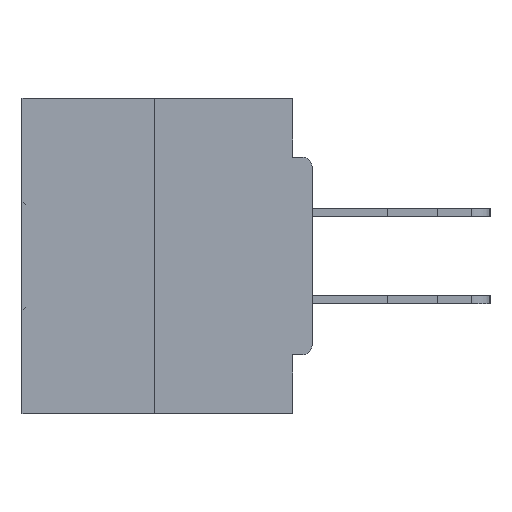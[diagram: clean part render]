
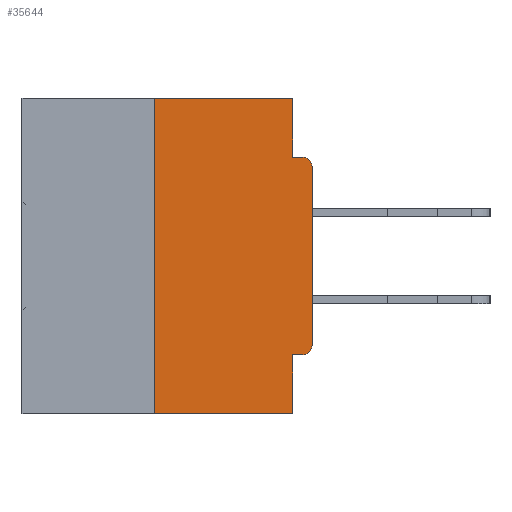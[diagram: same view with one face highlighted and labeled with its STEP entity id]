
A CAD part, left-side view. The second image highlights one B-rep face of the part: STEP entity #35644.
In plain terms, the highlighted planar face has unit normal (-1, 0, 0).
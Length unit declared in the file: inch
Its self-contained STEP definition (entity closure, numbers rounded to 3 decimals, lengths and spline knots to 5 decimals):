
#407 = VECTOR ( 'NONE', #23579, 39.37008 ) ;
#634 = DIRECTION ( 'NONE',  ( 1., 0., 0. ) ) ;
#1143 = EDGE_CURVE ( 'NONE', #27510, #11333, #8660, .T. ) ;
#1648 = CIRCLE ( 'NONE', #36667, 0.015 ) ;
#2024 = CARTESIAN_POINT ( 'NONE',  ( 0., 0.46, -0.5 ) ) ;
#2041 = ORIENTED_EDGE ( 'NONE', *, *, #32942, .F. ) ;
#2618 = VECTOR ( 'NONE', #38371, 39.37008 ) ;
#3004 = CARTESIAN_POINT ( 'NONE',  ( 0., 0.031, 0. ) ) ;
#3270 = CARTESIAN_POINT ( 'NONE',  ( 0., 0.015, -0.1085 ) ) ;
#3577 = ORIENTED_EDGE ( 'NONE', *, *, #40336, .F. ) ;
#3585 = DIRECTION ( 'NONE',  ( 0., 0., -1. ) ) ;
#3867 = VECTOR ( 'NONE', #13596, 39.37008 ) ;
#3952 = ORIENTED_EDGE ( 'NONE', *, *, #7599, .T. ) ;
#4136 = ORIENTED_EDGE ( 'NONE', *, *, #6865, .T. ) ;
#4516 = CARTESIAN_POINT ( 'NONE',  ( 0., 0., -0.4065 ) ) ;
#5076 = CARTESIAN_POINT ( 'NONE',  ( 0., 0., -0.3915 ) ) ;
#5557 = VERTEX_POINT ( 'NONE', #20639 ) ;
#6226 = ORIENTED_EDGE ( 'NONE', *, *, #40647, .T. ) ;
#6865 = EDGE_CURVE ( 'NONE', #42067, #28678, #41140, .T. ) ;
#7599 = EDGE_CURVE ( 'NONE', #28678, #8793, #22742, .T. ) ;
#7859 = FACE_OUTER_BOUND ( 'NONE', #12061, .T. ) ;
#8660 = LINE ( 'NONE', #38737, #43380 ) ;
#8755 = CARTESIAN_POINT ( 'NONE',  ( 0., 0., 0. ) ) ;
#8793 = VERTEX_POINT ( 'NONE', #30730 ) ;
#9559 = ORIENTED_EDGE ( 'NONE', *, *, #23249, .F. ) ;
#11333 = VERTEX_POINT ( 'NONE', #27280 ) ;
#12061 = EDGE_LOOP ( 'NONE', ( #13271, #2041, #13463, #39739, #3577, #4136, #3952, #6226, #15890, #9559 ) ) ;
#13271 = ORIENTED_EDGE ( 'NONE', *, *, #25175, .F. ) ;
#13463 = ORIENTED_EDGE ( 'NONE', *, *, #41080, .T. ) ;
#13570 = LINE ( 'NONE', #23430, #407 ) ;
#13596 = DIRECTION ( 'NONE',  ( 0., -1., 0. ) ) ;
#14031 = VECTOR ( 'NONE', #30005, 39.37008 ) ;
#14272 = CARTESIAN_POINT ( 'NONE',  ( 0., 0.015, -0.4065 ) ) ;
#15031 = VECTOR ( 'NONE', #28635, 39.37008 ) ;
#15579 = CARTESIAN_POINT ( 'NONE',  ( 0., 0.031, -0.0935 ) ) ;
#15890 = ORIENTED_EDGE ( 'NONE', *, *, #37789, .F. ) ;
#17876 = PLANE ( 'NONE',  #18477 ) ;
#18142 = LINE ( 'NONE', #23672, #3867 ) ;
#18477 = AXIS2_PLACEMENT_3D ( 'NONE', #34389, #634, #37721 ) ;
#18566 = CARTESIAN_POINT ( 'NONE',  ( 0., 0.031, -0.4065 ) ) ;
#18867 = AXIS2_PLACEMENT_3D ( 'NONE', #38060, #25012, #31910 ) ;
#20639 = CARTESIAN_POINT ( 'NONE',  ( 0., 0.25, 0. ) ) ;
#21188 = DIRECTION ( 'NONE',  ( -1., 0., 0. ) ) ;
#22742 = LINE ( 'NONE', #8755, #2618 ) ;
#23249 = EDGE_CURVE ( 'NONE', #31481, #32759, #34640, .T. ) ;
#23430 = CARTESIAN_POINT ( 'NONE',  ( 0., 0.25, 0. ) ) ;
#23579 = DIRECTION ( 'NONE',  ( 0., 0., 1. ) ) ;
#23672 = CARTESIAN_POINT ( 'NONE',  ( 0., 0.46, 0. ) ) ;
#25012 = DIRECTION ( 'NONE',  ( -1., 0., 0. ) ) ;
#25175 = EDGE_CURVE ( 'NONE', #5557, #31481, #18142, .T. ) ;
#26498 = LINE ( 'NONE', #4516, #39584 ) ;
#27280 = CARTESIAN_POINT ( 'NONE',  ( 0., 0.031, -0.5 ) ) ;
#27510 = VERTEX_POINT ( 'NONE', #18566 ) ;
#27581 = VERTEX_POINT ( 'NONE', #27611 ) ;
#27611 = CARTESIAN_POINT ( 'NONE',  ( 0., 0.015, -0.0935 ) ) ;
#28147 = DIRECTION ( 'NONE',  ( 0., 1., 0. ) ) ;
#28242 = DIRECTION ( 'NONE',  ( 0., 0., -1. ) ) ;
#28635 = DIRECTION ( 'NONE',  ( 0., -1., 0. ) ) ;
#28678 = VERTEX_POINT ( 'NONE', #5076 ) ;
#29885 = VECTOR ( 'NONE', #38340, 39.37008 ) ;
#30005 = DIRECTION ( 'NONE',  ( 0., 0., -1. ) ) ;
#30339 = LINE ( 'NONE', #2024, #15031 ) ;
#30730 = CARTESIAN_POINT ( 'NONE',  ( 0., 0., -0.1085 ) ) ;
#31481 = VERTEX_POINT ( 'NONE', #36552 ) ;
#31910 = DIRECTION ( 'NONE',  ( 0., 0., -1. ) ) ;
#32759 = VERTEX_POINT ( 'NONE', #15579 ) ;
#32942 = EDGE_CURVE ( 'NONE', #38615, #5557, #13570, .T. ) ;
#34389 = CARTESIAN_POINT ( 'NONE',  ( 0., 0.46, 0. ) ) ;
#34640 = LINE ( 'NONE', #3004, #14031 ) ;
#35644 = ADVANCED_FACE ( 'NONE', ( #7859 ), #17876, .F. ) ;
#36552 = CARTESIAN_POINT ( 'NONE',  ( 0., 0.031, 0. ) ) ;
#36667 = AXIS2_PLACEMENT_3D ( 'NONE', #3270, #21188, #3585 ) ;
#37721 = DIRECTION ( 'NONE',  ( 0., 0., -1. ) ) ;
#37789 = EDGE_CURVE ( 'NONE', #32759, #27581, #41391, .T. ) ;
#38060 = CARTESIAN_POINT ( 'NONE',  ( 0., 0.015, -0.3915 ) ) ;
#38340 = DIRECTION ( 'NONE',  ( 0., -1., 0. ) ) ;
#38371 = DIRECTION ( 'NONE',  ( 0., 0., 1. ) ) ;
#38615 = VERTEX_POINT ( 'NONE', #39921 ) ;
#38737 = CARTESIAN_POINT ( 'NONE',  ( 0., 0.031, -0.5 ) ) ;
#39584 = VECTOR ( 'NONE', #28147, 39.37008 ) ;
#39739 = ORIENTED_EDGE ( 'NONE', *, *, #1143, .F. ) ;
#39921 = CARTESIAN_POINT ( 'NONE',  ( 0., 0.25, -0.5 ) ) ;
#40336 = EDGE_CURVE ( 'NONE', #42067, #27510, #26498, .T. ) ;
#40647 = EDGE_CURVE ( 'NONE', #8793, #27581, #1648, .T. ) ;
#41080 = EDGE_CURVE ( 'NONE', #38615, #11333, #30339, .T. ) ;
#41092 = CARTESIAN_POINT ( 'NONE',  ( 0., 0., -0.0935 ) ) ;
#41140 = CIRCLE ( 'NONE', #18867, 0.015 ) ;
#41391 = LINE ( 'NONE', #41092, #29885 ) ;
#42067 = VERTEX_POINT ( 'NONE', #14272 ) ;
#43380 = VECTOR ( 'NONE', #28242, 39.37008 ) ;
